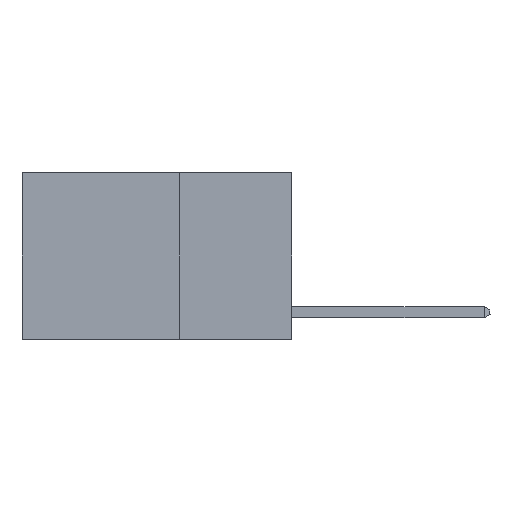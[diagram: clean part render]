
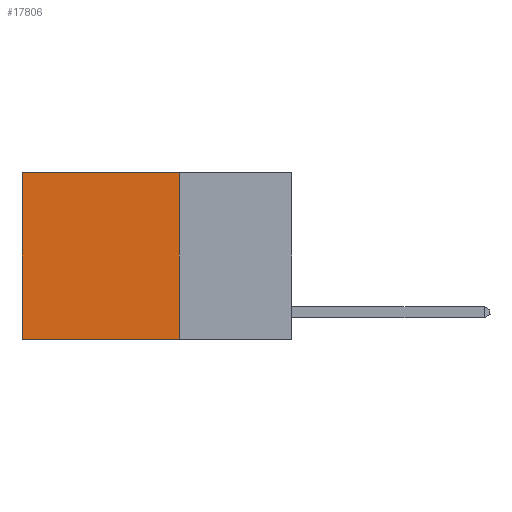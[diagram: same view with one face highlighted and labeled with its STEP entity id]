
A CAD part, left-side view. The second image highlights one B-rep face of the part: STEP entity #17806.
In plain terms, the highlighted planar face has unit normal (-1, 0, 0).
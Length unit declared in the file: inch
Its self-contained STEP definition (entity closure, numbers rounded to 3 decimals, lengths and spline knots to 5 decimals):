
#539 = CARTESIAN_POINT ( 'NONE',  ( 0.2625, 0.6, -0.37 ) ) ;
#608 = PLANE ( 'NONE',  #24018 ) ;
#864 = ORIENTED_EDGE ( 'NONE', *, *, #9268, .T. ) ;
#1024 = LINE ( 'NONE', #16795, #7368 ) ;
#1246 = CARTESIAN_POINT ( 'NONE',  ( 0.2625, 0.25, -0.37 ) ) ;
#1560 = VECTOR ( 'NONE', #19819, 39.37008 ) ;
#2520 = EDGE_CURVE ( 'NONE', #10089, #17494, #1024, .T. ) ;
#5020 = DIRECTION ( 'NONE',  ( 0., 1., 0. ) ) ;
#5147 = CARTESIAN_POINT ( 'NONE',  ( 0.2625, 0.6, 0. ) ) ;
#5781 = ORIENTED_EDGE ( 'NONE', *, *, #2520, .T. ) ;
#6362 = DIRECTION ( 'NONE',  ( 0., 0., -1. ) ) ;
#7368 = VECTOR ( 'NONE', #5020, 39.37008 ) ;
#8257 = FACE_OUTER_BOUND ( 'NONE', #21376, .T. ) ;
#8483 = CARTESIAN_POINT ( 'NONE',  ( 0.2625, 0.25, 0. ) ) ;
#8577 = LINE ( 'NONE', #14393, #20799 ) ;
#8812 = ORIENTED_EDGE ( 'NONE', *, *, #17151, .F. ) ;
#9268 = EDGE_CURVE ( 'NONE', #17494, #23217, #8577, .T. ) ;
#10066 = DIRECTION ( 'NONE',  ( 1., 0., 0. ) ) ;
#10089 = VERTEX_POINT ( 'NONE', #8483 ) ;
#12008 = CARTESIAN_POINT ( 'NONE',  ( 0.2625, 0.25, 0. ) ) ;
#12914 = ORIENTED_EDGE ( 'NONE', *, *, #13248, .F. ) ;
#13248 = EDGE_CURVE ( 'NONE', #10089, #20756, #21384, .T. ) ;
#14393 = CARTESIAN_POINT ( 'NONE',  ( 0.2625, 0.6, 0. ) ) ;
#16124 = DIRECTION ( 'NONE',  ( 0., 0., -1. ) ) ;
#16795 = CARTESIAN_POINT ( 'NONE',  ( 0.2625, 0.25, 0. ) ) ;
#17151 = EDGE_CURVE ( 'NONE', #20756, #23217, #24221, .T. ) ;
#17494 = VERTEX_POINT ( 'NONE', #5147 ) ;
#17806 = ADVANCED_FACE ( 'NONE', ( #8257 ), #608, .F. ) ;
#19819 = DIRECTION ( 'NONE',  ( 0., 0., -1. ) ) ;
#19946 = CARTESIAN_POINT ( 'NONE',  ( 0.2625, 0.25, 0. ) ) ;
#20338 = DIRECTION ( 'NONE',  ( 0., 1., 0. ) ) ;
#20756 = VERTEX_POINT ( 'NONE', #1246 ) ;
#20799 = VECTOR ( 'NONE', #6362, 39.37008 ) ;
#21376 = EDGE_LOOP ( 'NONE', ( #864, #8812, #12914, #5781 ) ) ;
#21384 = LINE ( 'NONE', #19946, #1560 ) ;
#22533 = CARTESIAN_POINT ( 'NONE',  ( 0.2625, 0.25, -0.37 ) ) ;
#23217 = VERTEX_POINT ( 'NONE', #539 ) ;
#23544 = VECTOR ( 'NONE', #20338, 39.37008 ) ;
#24018 = AXIS2_PLACEMENT_3D ( 'NONE', #12008, #10066, #16124 ) ;
#24221 = LINE ( 'NONE', #22533, #23544 ) ;
